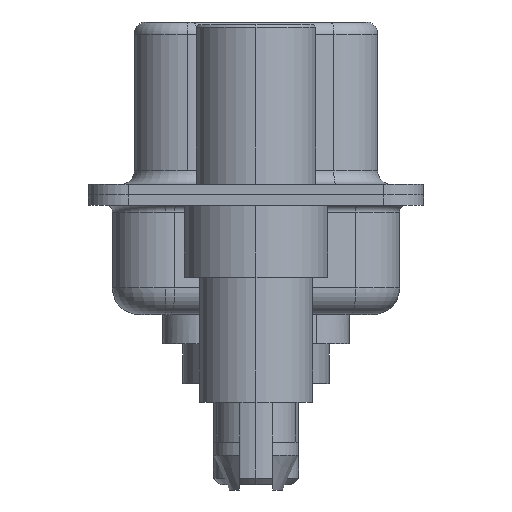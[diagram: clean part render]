
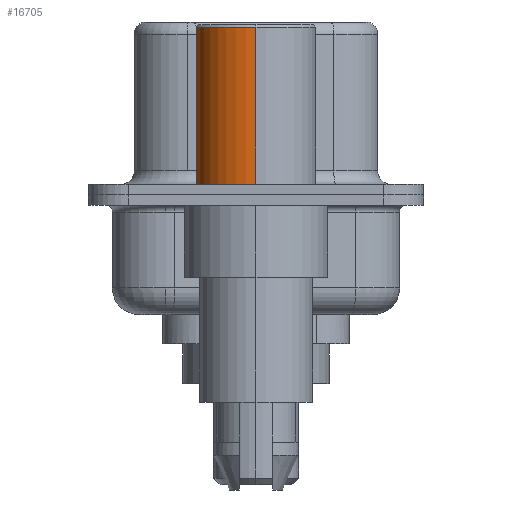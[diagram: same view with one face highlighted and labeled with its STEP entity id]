
A CAD part, left-side view. The second image highlights one B-rep face of the part: STEP entity #16705.
In plain terms, the highlighted cylindrical face has radius 2.25 mm (diameter 4.5 mm), a partial arc.
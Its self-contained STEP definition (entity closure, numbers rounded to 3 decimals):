
#340 = VECTOR ( 'NONE', #7173, 1000. ) ;
#1273 = CARTESIAN_POINT ( 'NONE',  ( 2.25, 0., 6.3 ) ) ;
#1323 = CARTESIAN_POINT ( 'NONE',  ( 0., 0., 6.3 ) ) ;
#1693 = VERTEX_POINT ( 'NONE', #1273 ) ;
#1839 = CARTESIAN_POINT ( 'NONE',  ( -2.25, 0., 0.581 ) ) ;
#2646 = DIRECTION ( 'NONE',  ( 0., 0., 1. ) ) ;
#3084 = CARTESIAN_POINT ( 'NONE',  ( -2.25, 0., 0.4 ) ) ;
#3231 = DIRECTION ( 'NONE',  ( 0., 0., 1. ) ) ;
#3344 = DIRECTION ( 'NONE',  ( 0., 0., 1. ) ) ;
#4015 = LINE ( 'NONE', #12675, #340 ) ;
#4227 = ORIENTED_EDGE ( 'NONE', *, *, #7659, .F. ) ;
#4413 = VERTEX_POINT ( 'NONE', #14925 ) ;
#4494 = ORIENTED_EDGE ( 'NONE', *, *, #14290, .T. ) ;
#4639 = EDGE_CURVE ( 'NONE', #1693, #5607, #13633, .T. ) ;
#4963 = DIRECTION ( 'NONE',  ( 0., 0., 1. ) ) ;
#5607 = VERTEX_POINT ( 'NONE', #7639 ) ;
#5819 = FACE_OUTER_BOUND ( 'NONE', #17476, .T. ) ;
#7173 = DIRECTION ( 'NONE',  ( 0., 0., 1. ) ) ;
#7280 = ORIENTED_EDGE ( 'NONE', *, *, #16489, .T. ) ;
#7639 = CARTESIAN_POINT ( 'NONE',  ( -2.25, 0., 6.3 ) ) ;
#7659 = EDGE_CURVE ( 'NONE', #4413, #1693, #4015, .T. ) ;
#7691 = CARTESIAN_POINT ( 'NONE',  ( 0., 0., 0.581 ) ) ;
#8002 = LINE ( 'NONE', #1839, #14938 ) ;
#8551 = AXIS2_PLACEMENT_3D ( 'NONE', #10918, #2646, #12291 ) ;
#9550 = CIRCLE ( 'NONE', #8551, 2.25 ) ;
#10819 = AXIS2_PLACEMENT_3D ( 'NONE', #7691, #4963, #14663 ) ;
#10918 = CARTESIAN_POINT ( 'NONE',  ( 0., 0., 0.4 ) ) ;
#11926 = AXIS2_PLACEMENT_3D ( 'NONE', #1323, #3344, #16007 ) ;
#12291 = DIRECTION ( 'NONE',  ( 1., 0., 0. ) ) ;
#12295 = CYLINDRICAL_SURFACE ( 'NONE', #10819, 2.25 ) ;
#12675 = CARTESIAN_POINT ( 'NONE',  ( 2.25, 0., 0.581 ) ) ;
#13062 = VERTEX_POINT ( 'NONE', #3084 ) ;
#13633 = CIRCLE ( 'NONE', #11926, 2.25 ) ;
#14290 = EDGE_CURVE ( 'NONE', #4413, #13062, #9550, .T. ) ;
#14663 = DIRECTION ( 'NONE',  ( 1., 0., 0. ) ) ;
#14925 = CARTESIAN_POINT ( 'NONE',  ( 2.25, 0., 0.4 ) ) ;
#14938 = VECTOR ( 'NONE', #3231, 1000. ) ;
#16007 = DIRECTION ( 'NONE',  ( 1., 0., 0. ) ) ;
#16489 = EDGE_CURVE ( 'NONE', #13062, #5607, #8002, .T. ) ;
#16705 = ADVANCED_FACE ( 'NONE', ( #5819 ), #12295, .T. ) ;
#17476 = EDGE_LOOP ( 'NONE', ( #4494, #7280, #17890, #4227 ) ) ;
#17890 = ORIENTED_EDGE ( 'NONE', *, *, #4639, .F. ) ;
